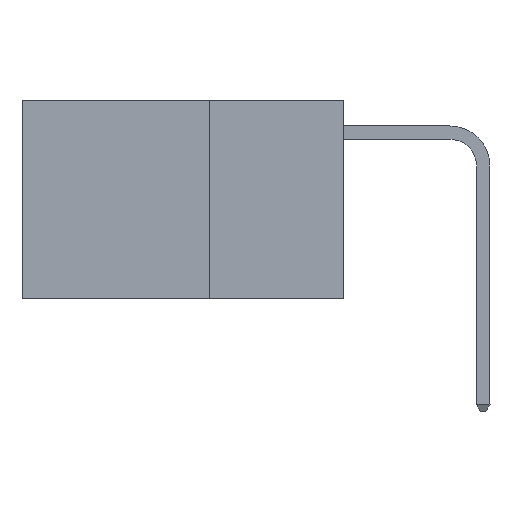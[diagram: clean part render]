
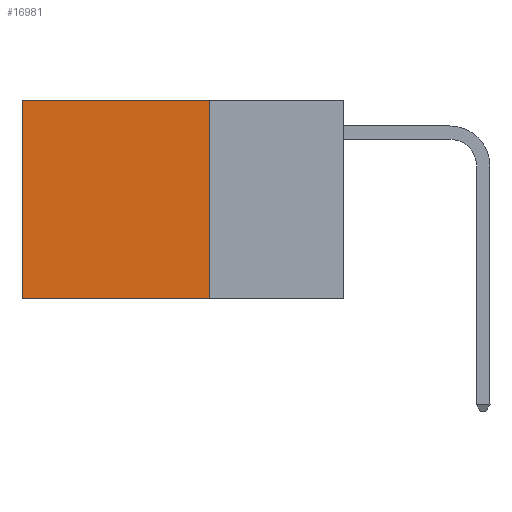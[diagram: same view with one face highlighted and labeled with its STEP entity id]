
A CAD part, left-side view. The second image highlights one B-rep face of the part: STEP entity #16981.
In plain terms, the highlighted planar face has unit normal (-1, 0, 0).
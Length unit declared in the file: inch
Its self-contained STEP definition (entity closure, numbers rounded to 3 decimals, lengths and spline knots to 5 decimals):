
#912 = CARTESIAN_POINT ( 'NONE',  ( 0.2625, 0.25, -0.37 ) ) ;
#3012 = VERTEX_POINT ( 'NONE', #18709 ) ;
#3321 = EDGE_CURVE ( 'NONE', #14357, #7009, #16167, .T. ) ;
#4207 = DIRECTION ( 'NONE',  ( 1., 0., 0. ) ) ;
#4525 = CARTESIAN_POINT ( 'NONE',  ( 0.2625, 0.25, 0. ) ) ;
#4850 = EDGE_LOOP ( 'NONE', ( #6931, #8148, #7059, #11659 ) ) ;
#5456 = VECTOR ( 'NONE', #15917, 39.37008 ) ;
#5474 = VECTOR ( 'NONE', #17538, 39.37008 ) ;
#5938 = CARTESIAN_POINT ( 'NONE',  ( 0.2625, 0.25, -0.37 ) ) ;
#6670 = EDGE_CURVE ( 'NONE', #3012, #14357, #9441, .T. ) ;
#6931 = ORIENTED_EDGE ( 'NONE', *, *, #3321, .T. ) ;
#7009 = VERTEX_POINT ( 'NONE', #16756 ) ;
#7059 = ORIENTED_EDGE ( 'NONE', *, *, #8364, .F. ) ;
#8148 = ORIENTED_EDGE ( 'NONE', *, *, #20356, .F. ) ;
#8364 = EDGE_CURVE ( 'NONE', #3012, #20124, #11209, .T. ) ;
#9441 = LINE ( 'NONE', #4525, #5474 ) ;
#9506 = LINE ( 'NONE', #5938, #5456 ) ;
#9875 = VECTOR ( 'NONE', #20461, 39.37008 ) ;
#11209 = LINE ( 'NONE', #12683, #9875 ) ;
#11659 = ORIENTED_EDGE ( 'NONE', *, *, #6670, .T. ) ;
#12683 = CARTESIAN_POINT ( 'NONE',  ( 0.2625, 0.25, 0. ) ) ;
#13033 = CARTESIAN_POINT ( 'NONE',  ( 0.2625, 0.6, 0. ) ) ;
#13114 = VECTOR ( 'NONE', #19436, 39.37008 ) ;
#13753 = CARTESIAN_POINT ( 'NONE',  ( 0.2625, 0.25, 0. ) ) ;
#13868 = DIRECTION ( 'NONE',  ( 0., 0., -1. ) ) ;
#14357 = VERTEX_POINT ( 'NONE', #19330 ) ;
#15022 = FACE_OUTER_BOUND ( 'NONE', #4850, .T. ) ;
#15413 = PLANE ( 'NONE',  #16140 ) ;
#15917 = DIRECTION ( 'NONE',  ( 0., 1., 0. ) ) ;
#16140 = AXIS2_PLACEMENT_3D ( 'NONE', #13753, #4207, #13868 ) ;
#16167 = LINE ( 'NONE', #13033, #13114 ) ;
#16756 = CARTESIAN_POINT ( 'NONE',  ( 0.2625, 0.6, -0.37 ) ) ;
#16981 = ADVANCED_FACE ( 'NONE', ( #15022 ), #15413, .F. ) ;
#17538 = DIRECTION ( 'NONE',  ( 0., 1., 0. ) ) ;
#18709 = CARTESIAN_POINT ( 'NONE',  ( 0.2625, 0.25, 0. ) ) ;
#19330 = CARTESIAN_POINT ( 'NONE',  ( 0.2625, 0.6, 0. ) ) ;
#19436 = DIRECTION ( 'NONE',  ( 0., 0., -1. ) ) ;
#20124 = VERTEX_POINT ( 'NONE', #912 ) ;
#20356 = EDGE_CURVE ( 'NONE', #20124, #7009, #9506, .T. ) ;
#20461 = DIRECTION ( 'NONE',  ( 0., 0., -1. ) ) ;
